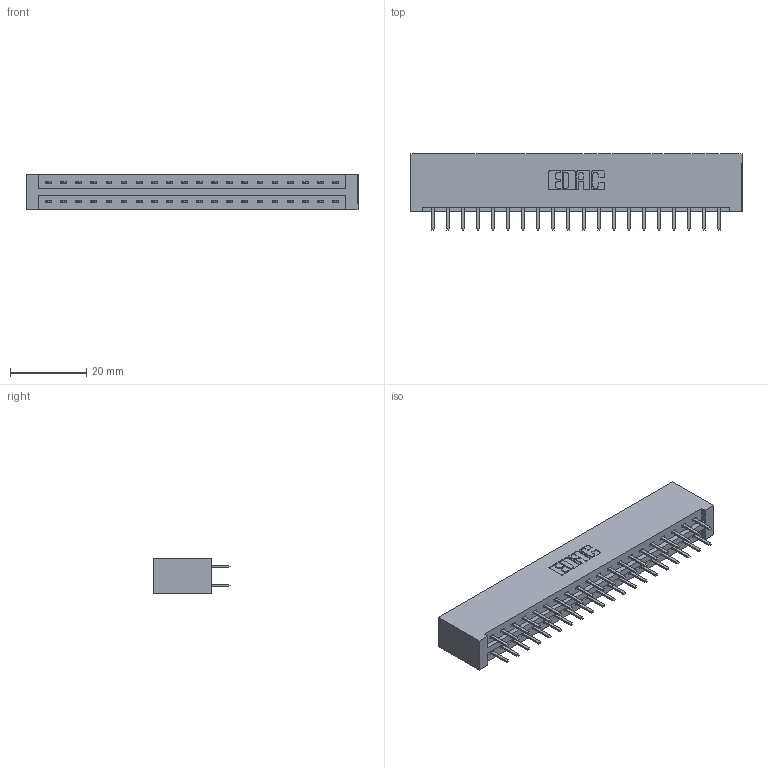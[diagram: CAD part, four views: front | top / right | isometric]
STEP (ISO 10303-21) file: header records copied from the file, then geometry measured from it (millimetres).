
FILE_DESCRIPTION (( 'STEP AP203' ), '1' );
FILE_NAME ('337-040-520-201.STEP', '2018-08-08T08:53:50', ( '' ), ( '' ), 'SwSTEP 2.0', 'SolidWorks 2016', '' );
FILE_SCHEMA (( 'CONFIG_CONTROL_DESIGN' ));
Length unit declared in the file: inch
Products named in the file (3): 337 Part_No Mounting Lugs; 345-292-001_345-293-120; 337-040-520-201
Assembly tree (41 placements, depth 2):
  337-040-520-201
    337 Part_No Mounting Lugs
    345-292-001_345-293-120  x40
Bounding box: 87.12 x 20.02 x 9.4 mm (x, y, z)
Volume: 9631.9 mm3; surface area: 10681.1 mm2
Topology: 41 solids, 41 shells, 2426 faces, 7047 edges, 4590 vertices
Faces by surface type: plane 1666, cylinder 760
Entity records: 18189 total; most frequent: CARTESIAN_POINT 3094, ORIENTED_EDGE 3018, DIRECTION 2653, EDGE_CURVE 1509, LINE 1385, VECTOR 1385, VERTEX_POINT 1002, AXIS2_PLACEMENT_3D 634
